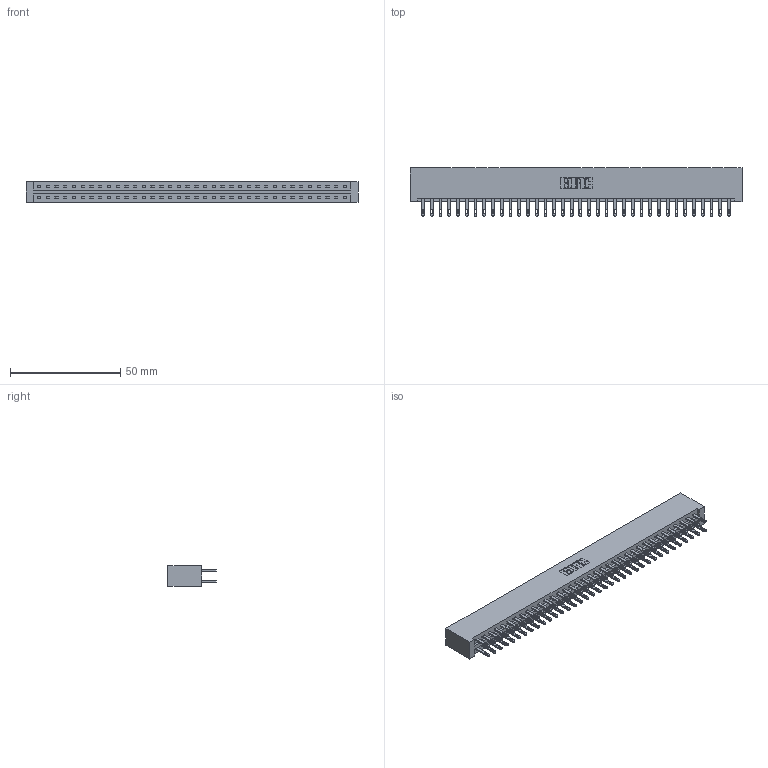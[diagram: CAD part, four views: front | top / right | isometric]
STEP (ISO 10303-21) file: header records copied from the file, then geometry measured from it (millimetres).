
FILE_DESCRIPTION (( 'STEP AP203' ), '1' );
FILE_NAME ('337-072-500-201.STEP', '2019-10-10T02:02:15', ( '' ), ( '' ), 'SwSTEP 2.0', 'SolidWorks 2016', '' );
FILE_SCHEMA (( 'CONFIG_CONTROL_DESIGN' ));
Length unit declared in the file: inch
Products named in the file (3): 345-292-001_345-293-100; 337-072-500-201; 337 Part_No Mounting Lugs
Assembly tree (73 placements, depth 2):
  337-072-500-201
    337 Part_No Mounting Lugs
    345-292-001_345-293-100  x72
Bounding box: 150.52 x 21.85 x 9.4 mm (x, y, z)
Volume: 16763.9 mm3; surface area: 19748.4 mm2
Topology: 73 solids, 73 shells, 3706 faces, 11303 edges, 7534 vertices
Faces by surface type: plane 2370, cylinder 1336
Entity records: 28341 total; most frequent: CARTESIAN_POINT 4778, ORIENTED_EDGE 4714, DIRECTION 4069, EDGE_CURVE 2357, VECTOR 2233, LINE 2233, VERTEX_POINT 1570, AXIS2_PLACEMENT_3D 918
